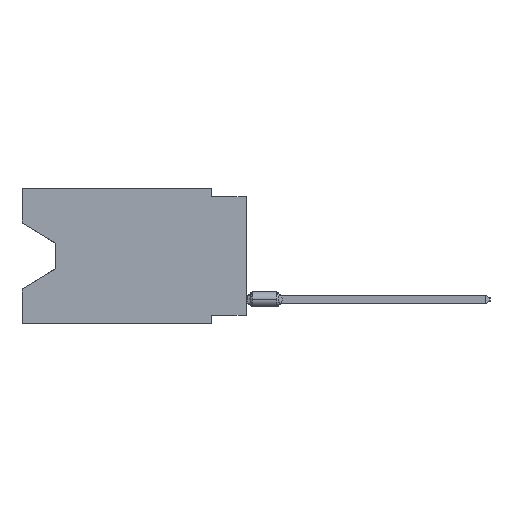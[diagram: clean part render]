
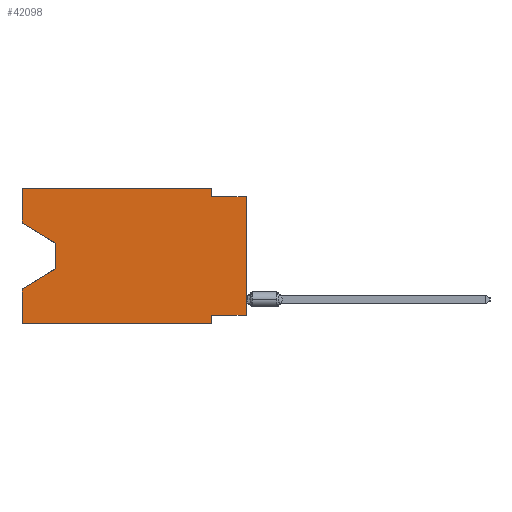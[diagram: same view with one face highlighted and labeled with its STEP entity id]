
A CAD part, left-side view. The second image highlights one B-rep face of the part: STEP entity #42098.
In plain terms, the highlighted planar face has unit normal (-1, 0, 0).
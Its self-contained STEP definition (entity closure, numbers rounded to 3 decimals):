
#11 = CARTESIAN_POINT ( 'NONE',  ( 0., 13.97, -5.893 ) ) ;
#2469 = CARTESIAN_POINT ( 'NONE',  ( 0., 2.54, -9.906 ) ) ;
#4413 = VERTEX_POINT ( 'NONE', #2469 ) ;
#7416 = EDGE_CURVE ( 'NONE', #48362, #4413, #42254, .T. ) ;
#7844 = ORIENTED_EDGE ( 'NONE', *, *, #27045, .F. ) ;
#9016 = LINE ( 'NONE', #54079, #18705 ) ;
#9299 = CARTESIAN_POINT ( 'NONE',  ( 0., 16.383, -2.546 ) ) ;
#9501 = AXIS2_PLACEMENT_3D ( 'NONE', #16025, #34325, #52655 ) ;
#12133 = EDGE_CURVE ( 'NONE', #17412, #43705, #9016, .T. ) ;
#12157 = DIRECTION ( 'NONE',  ( 0., 0., 1. ) ) ;
#12891 = CARTESIAN_POINT ( 'NONE',  ( 0., 0., -9.271 ) ) ;
#12913 = DIRECTION ( 'NONE',  ( 0., 0., 1. ) ) ;
#13553 = VECTOR ( 'NONE', #17720, 1000. ) ;
#14004 = EDGE_CURVE ( 'NONE', #47053, #51613, #35913, .T. ) ;
#14986 = VECTOR ( 'NONE', #12913, 1000. ) ;
#15205 = CARTESIAN_POINT ( 'NONE',  ( 0., 2.54, 0. ) ) ;
#15576 = CARTESIAN_POINT ( 'NONE',  ( 0., 13.97, -5.893 ) ) ;
#15989 = ORIENTED_EDGE ( 'NONE', *, *, #31138, .T. ) ;
#16025 = CARTESIAN_POINT ( 'NONE',  ( 0., 16.383, 0. ) ) ;
#17335 = ORIENTED_EDGE ( 'NONE', *, *, #12133, .F. ) ;
#17412 = VERTEX_POINT ( 'NONE', #21444 ) ;
#17720 = DIRECTION ( 'NONE',  ( 0., 0., -1. ) ) ;
#17945 = EDGE_CURVE ( 'NONE', #17412, #20665, #23436, .T. ) ;
#18074 = ORIENTED_EDGE ( 'NONE', *, *, #32392, .F. ) ;
#18131 = ORIENTED_EDGE ( 'NONE', *, *, #14004, .F. ) ;
#18330 = DIRECTION ( 'NONE',  ( 0., 0.855, -0.519 ) ) ;
#18705 = VECTOR ( 'NONE', #45630, 1000. ) ;
#18962 = CARTESIAN_POINT ( 'NONE',  ( 0., 2.54, -0.635 ) ) ;
#19043 = DIRECTION ( 'NONE',  ( 0., 0., -1. ) ) ;
#20288 = LINE ( 'NONE', #44263, #34551 ) ;
#20307 = DIRECTION ( 'NONE',  ( 0., -1., 0. ) ) ;
#20381 = LINE ( 'NONE', #25193, #50700 ) ;
#20665 = VERTEX_POINT ( 'NONE', #27692 ) ;
#20834 = ORIENTED_EDGE ( 'NONE', *, *, #56916, .F. ) ;
#21444 = CARTESIAN_POINT ( 'NONE',  ( 0., 16.383, -2.546 ) ) ;
#21755 = ORIENTED_EDGE ( 'NONE', *, *, #17945, .T. ) ;
#21843 = VECTOR ( 'NONE', #27338, 1000. ) ;
#22943 = CARTESIAN_POINT ( 'NONE',  ( 0., 16.383, -9.906 ) ) ;
#23436 = LINE ( 'NONE', #9299, #21843 ) ;
#23561 = LINE ( 'NONE', #42150, #40320 ) ;
#23677 = LINE ( 'NONE', #41681, #24967 ) ;
#24967 = VECTOR ( 'NONE', #50394, 1000. ) ;
#25180 = ORIENTED_EDGE ( 'NONE', *, *, #56230, .T. ) ;
#25193 = CARTESIAN_POINT ( 'NONE',  ( 0., 16.383, 0. ) ) ;
#26136 = LINE ( 'NONE', #57341, #14986 ) ;
#26991 = EDGE_LOOP ( 'NONE', ( #21755, #25180, #31872, #18074, #15989, #30332, #7844, #40714, #18131, #20834, #35113, #17335 ) ) ;
#27045 = EDGE_CURVE ( 'NONE', #58613, #48362, #23677, .T. ) ;
#27338 = DIRECTION ( 'NONE',  ( 0., -0.855, -0.519 ) ) ;
#27692 = CARTESIAN_POINT ( 'NONE',  ( 0., 13.97, -4.013 ) ) ;
#27922 = VECTOR ( 'NONE', #56072, 1000. ) ;
#29272 = VERTEX_POINT ( 'NONE', #15576 ) ;
#30293 = VECTOR ( 'NONE', #20307, 1000. ) ;
#30332 = ORIENTED_EDGE ( 'NONE', *, *, #7416, .F. ) ;
#31138 = EDGE_CURVE ( 'NONE', #32984, #4413, #47021, .T. ) ;
#31872 = ORIENTED_EDGE ( 'NONE', *, *, #54211, .T. ) ;
#31925 = VECTOR ( 'NONE', #36201, 1000. ) ;
#32392 = EDGE_CURVE ( 'NONE', #32984, #35638, #26136, .T. ) ;
#32410 = LINE ( 'NONE', #11, #50297 ) ;
#32984 = VERTEX_POINT ( 'NONE', #22943 ) ;
#33903 = CARTESIAN_POINT ( 'NONE',  ( 0., 2.54, -9.271 ) ) ;
#34307 = EDGE_CURVE ( 'NONE', #43705, #47634, #20381, .T. ) ;
#34325 = DIRECTION ( 'NONE',  ( 1., 0., 0. ) ) ;
#34551 = VECTOR ( 'NONE', #12157, 1000. ) ;
#35113 = ORIENTED_EDGE ( 'NONE', *, *, #34307, .F. ) ;
#35638 = VERTEX_POINT ( 'NONE', #52041 ) ;
#35913 = LINE ( 'NONE', #54240, #31925 ) ;
#36201 = DIRECTION ( 'NONE',  ( 0., -1., 0. ) ) ;
#38843 = FACE_OUTER_BOUND ( 'NONE', #26991, .T. ) ;
#39262 = DIRECTION ( 'NONE',  ( 0., -1., 0. ) ) ;
#39363 = CARTESIAN_POINT ( 'NONE',  ( 0., 2.54, 0. ) ) ;
#40320 = VECTOR ( 'NONE', #19043, 1000. ) ;
#40714 = ORIENTED_EDGE ( 'NONE', *, *, #50460, .T. ) ;
#41681 = CARTESIAN_POINT ( 'NONE',  ( 0., 0., -9.271 ) ) ;
#42098 = ADVANCED_FACE ( 'NONE', ( #38843 ), #57167, .F. ) ;
#42150 = CARTESIAN_POINT ( 'NONE',  ( 0., 13.97, -4.013 ) ) ;
#42254 = LINE ( 'NONE', #55783, #27922 ) ;
#43705 = VERTEX_POINT ( 'NONE', #53611 ) ;
#44263 = CARTESIAN_POINT ( 'NONE',  ( 0., 0., 0. ) ) ;
#44274 = CARTESIAN_POINT ( 'NONE',  ( 0., 0., -0.635 ) ) ;
#45630 = DIRECTION ( 'NONE',  ( 0., 0., 1. ) ) ;
#47021 = LINE ( 'NONE', #51227, #30293 ) ;
#47053 = VERTEX_POINT ( 'NONE', #18962 ) ;
#47634 = VERTEX_POINT ( 'NONE', #15205 ) ;
#48362 = VERTEX_POINT ( 'NONE', #33903 ) ;
#49259 = LINE ( 'NONE', #39363, #13553 ) ;
#50297 = VECTOR ( 'NONE', #18330, 1000. ) ;
#50394 = DIRECTION ( 'NONE',  ( 0., 1., 0. ) ) ;
#50460 = EDGE_CURVE ( 'NONE', #58613, #51613, #20288, .T. ) ;
#50700 = VECTOR ( 'NONE', #39262, 1000. ) ;
#51227 = CARTESIAN_POINT ( 'NONE',  ( 0., 16.383, -9.906 ) ) ;
#51613 = VERTEX_POINT ( 'NONE', #44274 ) ;
#52041 = CARTESIAN_POINT ( 'NONE',  ( 0., 16.383, -7.36 ) ) ;
#52655 = DIRECTION ( 'NONE',  ( 0., 0., -1. ) ) ;
#53611 = CARTESIAN_POINT ( 'NONE',  ( 0., 16.383, 0. ) ) ;
#54079 = CARTESIAN_POINT ( 'NONE',  ( 0., 16.383, 0. ) ) ;
#54211 = EDGE_CURVE ( 'NONE', #29272, #35638, #32410, .T. ) ;
#54240 = CARTESIAN_POINT ( 'NONE',  ( 0., 0., -0.635 ) ) ;
#55783 = CARTESIAN_POINT ( 'NONE',  ( 0., 2.54, -9.906 ) ) ;
#56072 = DIRECTION ( 'NONE',  ( 0., 0., -1. ) ) ;
#56230 = EDGE_CURVE ( 'NONE', #20665, #29272, #23561, .T. ) ;
#56916 = EDGE_CURVE ( 'NONE', #47634, #47053, #49259, .T. ) ;
#57167 = PLANE ( 'NONE',  #9501 ) ;
#57341 = CARTESIAN_POINT ( 'NONE',  ( 0., 16.383, 0. ) ) ;
#58613 = VERTEX_POINT ( 'NONE', #12891 ) ;
